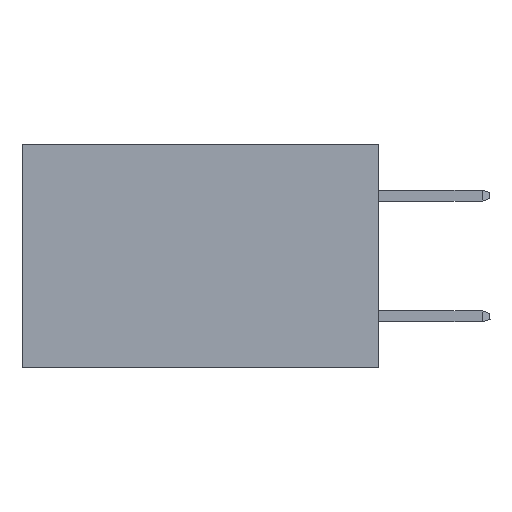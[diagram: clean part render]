
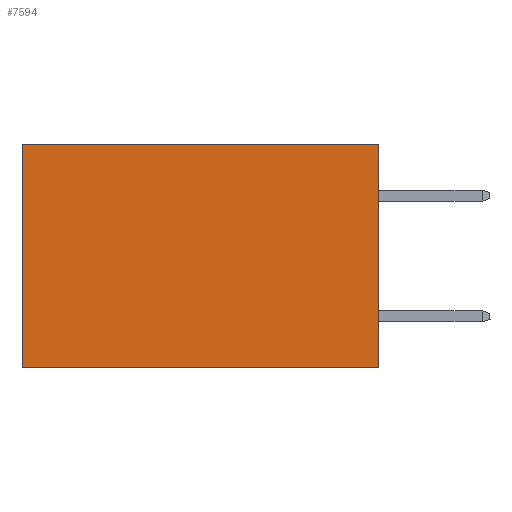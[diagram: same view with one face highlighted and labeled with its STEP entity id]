
A CAD part, left-side view. The second image highlights one B-rep face of the part: STEP entity #7594.
In plain terms, the highlighted planar face has unit normal (-1, 0, 0).
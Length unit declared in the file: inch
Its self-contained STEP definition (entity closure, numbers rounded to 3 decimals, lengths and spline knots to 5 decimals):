
#475 = EDGE_LOOP ( 'NONE', ( #6360, #24397, #16485, #10312 ) ) ;
#2935 = VERTEX_POINT ( 'NONE', #17357 ) ;
#4458 = LINE ( 'NONE', #25949, #25312 ) ;
#5599 = CARTESIAN_POINT ( 'NONE',  ( 0.277, 0., -0.37 ) ) ;
#5742 = VECTOR ( 'NONE', #12761, 39.37008 ) ;
#5860 = LINE ( 'NONE', #18043, #10716 ) ;
#6360 = ORIENTED_EDGE ( 'NONE', *, *, #20869, .T. ) ;
#7594 = ADVANCED_FACE ( 'NONE', ( #13068 ), #22371, .F. ) ;
#8365 = EDGE_CURVE ( 'NONE', #17833, #21339, #26178, .T. ) ;
#10147 = DIRECTION ( 'NONE',  ( 0., 0., -1. ) ) ;
#10312 = ORIENTED_EDGE ( 'NONE', *, *, #8365, .T. ) ;
#10716 = VECTOR ( 'NONE', #10147, 39.37008 ) ;
#10759 = CARTESIAN_POINT ( 'NONE',  ( 0.277, 0.59, -0.37 ) ) ;
#10839 = VECTOR ( 'NONE', #14537, 39.37008 ) ;
#11229 = LINE ( 'NONE', #10759, #5742 ) ;
#11946 = CARTESIAN_POINT ( 'NONE',  ( 0.277, 0.59, 0. ) ) ;
#12761 = DIRECTION ( 'NONE',  ( 0., 0., -1. ) ) ;
#12796 = AXIS2_PLACEMENT_3D ( 'NONE', #21654, #21263, #20784 ) ;
#13068 = FACE_OUTER_BOUND ( 'NONE', #475, .T. ) ;
#13797 = EDGE_CURVE ( 'NONE', #17833, #21280, #5860, .T. ) ;
#14537 = DIRECTION ( 'NONE',  ( 0., 1., 0. ) ) ;
#14686 = CARTESIAN_POINT ( 'NONE',  ( 0.277, 0., 0. ) ) ;
#15902 = DIRECTION ( 'NONE',  ( 0., 1., 0. ) ) ;
#16485 = ORIENTED_EDGE ( 'NONE', *, *, #13797, .F. ) ;
#17357 = CARTESIAN_POINT ( 'NONE',  ( 0.277, 0.59, -0.37 ) ) ;
#17833 = VERTEX_POINT ( 'NONE', #25971 ) ;
#18043 = CARTESIAN_POINT ( 'NONE',  ( 0.277, 0., -0.37 ) ) ;
#20784 = DIRECTION ( 'NONE',  ( 0., 0., -1. ) ) ;
#20869 = EDGE_CURVE ( 'NONE', #21339, #2935, #11229, .T. ) ;
#21263 = DIRECTION ( 'NONE',  ( 1., 0., 0. ) ) ;
#21280 = VERTEX_POINT ( 'NONE', #5599 ) ;
#21339 = VERTEX_POINT ( 'NONE', #11946 ) ;
#21342 = EDGE_CURVE ( 'NONE', #21280, #2935, #4458, .T. ) ;
#21654 = CARTESIAN_POINT ( 'NONE',  ( 0.277, 0., -0.37 ) ) ;
#22371 = PLANE ( 'NONE',  #12796 ) ;
#24397 = ORIENTED_EDGE ( 'NONE', *, *, #21342, .F. ) ;
#25312 = VECTOR ( 'NONE', #15902, 39.37008 ) ;
#25949 = CARTESIAN_POINT ( 'NONE',  ( 0.277, 0., -0.37 ) ) ;
#25971 = CARTESIAN_POINT ( 'NONE',  ( 0.277, 0., 0. ) ) ;
#26178 = LINE ( 'NONE', #14686, #10839 ) ;
